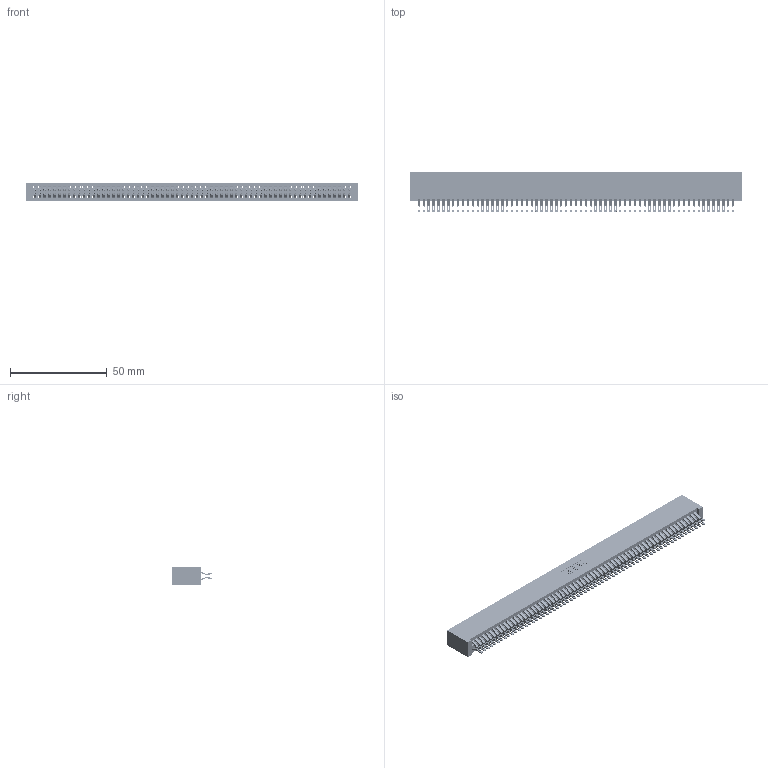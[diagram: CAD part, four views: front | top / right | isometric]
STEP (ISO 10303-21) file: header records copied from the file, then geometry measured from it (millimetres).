
FILE_DESCRIPTION (( 'STEP AP203' ), '1' );
FILE_NAME ('345-130-555-201.STEP', '2018-10-20T01:18:42', ( '' ), ( '' ), 'SwSTEP 2.0', 'SolidWorks 2016', '' );
FILE_SCHEMA (( 'CONFIG_CONTROL_DESIGN' ));
Length unit declared in the file: inch
Products named in the file (3): 345-292-001_555 Tail; 345 Part_No Mounting Lugs; 345-130-555-201
Assembly tree (131 placements, depth 2):
  345-130-555-201
    345 Part_No Mounting Lugs
    345-292-001_555 Tail  x130
Bounding box: 171.7 x 21.13 x 9.4 mm (x, y, z)
Volume: 17886 mm3; surface area: 28498.7 mm2
Topology: 131 solids, 131 shells, 7398 faces, 23327 edges, 15550 vertices
Faces by surface type: plane 4106, cylinder 3292
Entity records: 47953 total; most frequent: CARTESIAN_POINT 8050, ORIENTED_EDGE 7954, DIRECTION 7033, EDGE_CURVE 3977, VECTOR 3573, LINE 3573, VERTEX_POINT 2650, AXIS2_PLACEMENT_3D 1730
